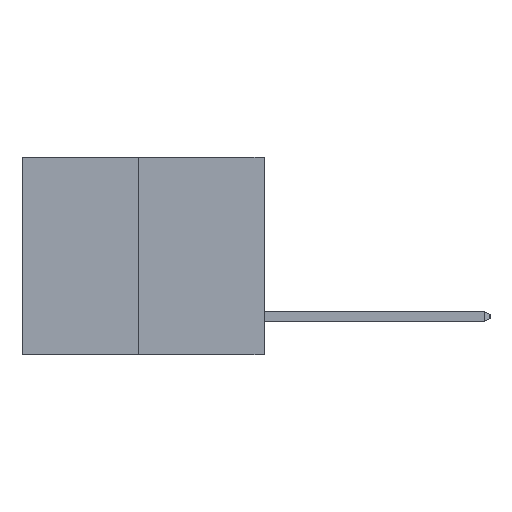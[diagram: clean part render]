
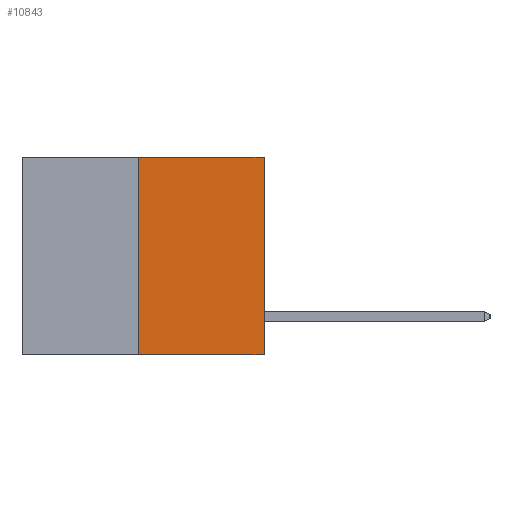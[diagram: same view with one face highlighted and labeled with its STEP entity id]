
A CAD part, left-side view. The second image highlights one B-rep face of the part: STEP entity #10843.
In plain terms, the highlighted planar face has unit normal (-1, 0, 0).
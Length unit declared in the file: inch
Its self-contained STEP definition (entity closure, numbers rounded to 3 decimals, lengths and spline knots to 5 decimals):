
#580 = LINE ( 'NONE', #10422, #9586 ) ;
#857 = CARTESIAN_POINT ( 'NONE',  ( 0., 0., 0. ) ) ;
#1157 = CARTESIAN_POINT ( 'NONE',  ( 0., 0.6, 0. ) ) ;
#1244 = CARTESIAN_POINT ( 'NONE',  ( 0., 0.312, -0.49 ) ) ;
#1453 = ORIENTED_EDGE ( 'NONE', *, *, #2829, .T. ) ;
#1583 = CARTESIAN_POINT ( 'NONE',  ( 0., 0., -0.49 ) ) ;
#1848 = FACE_OUTER_BOUND ( 'NONE', #2787, .T. ) ;
#2077 = CARTESIAN_POINT ( 'NONE',  ( 0., 0.6, -0.49 ) ) ;
#2404 = PLANE ( 'NONE',  #6178 ) ;
#2787 = EDGE_LOOP ( 'NONE', ( #13172, #1453, #3971, #11231 ) ) ;
#2829 = EDGE_CURVE ( 'NONE', #10470, #15645, #11234, .T. ) ;
#3025 = DIRECTION ( 'NONE',  ( 0., 0., 1. ) ) ;
#3500 = DIRECTION ( 'NONE',  ( 0., -1., 0. ) ) ;
#3876 = VERTEX_POINT ( 'NONE', #857 ) ;
#3971 = ORIENTED_EDGE ( 'NONE', *, *, #5435, .T. ) ;
#4559 = CARTESIAN_POINT ( 'NONE',  ( 0., 0.6, 0. ) ) ;
#5435 = EDGE_CURVE ( 'NONE', #15645, #3876, #580, .T. ) ;
#6178 = AXIS2_PLACEMENT_3D ( 'NONE', #1157, #14856, #16010 ) ;
#6462 = DIRECTION ( 'NONE',  ( 0., 0., 1. ) ) ;
#6846 = CARTESIAN_POINT ( 'NONE',  ( 0., 0.312, 0. ) ) ;
#7126 = CARTESIAN_POINT ( 'NONE',  ( 0., 0.312, -0.49 ) ) ;
#8089 = EDGE_CURVE ( 'NONE', #12696, #3876, #8664, .T. ) ;
#8664 = LINE ( 'NONE', #4559, #17399 ) ;
#9586 = VECTOR ( 'NONE', #6462, 39.37008 ) ;
#10257 = DIRECTION ( 'NONE',  ( 0., -1., 0. ) ) ;
#10382 = VECTOR ( 'NONE', #3500, 39.37008 ) ;
#10422 = CARTESIAN_POINT ( 'NONE',  ( 0., 0., 0. ) ) ;
#10470 = VERTEX_POINT ( 'NONE', #7126 ) ;
#10843 = ADVANCED_FACE ( 'NONE', ( #1848 ), #2404, .F. ) ;
#11231 = ORIENTED_EDGE ( 'NONE', *, *, #8089, .F. ) ;
#11234 = LINE ( 'NONE', #2077, #10382 ) ;
#12696 = VERTEX_POINT ( 'NONE', #6846 ) ;
#12871 = LINE ( 'NONE', #1244, #16032 ) ;
#13172 = ORIENTED_EDGE ( 'NONE', *, *, #14270, .F. ) ;
#14270 = EDGE_CURVE ( 'NONE', #10470, #12696, #12871, .T. ) ;
#14856 = DIRECTION ( 'NONE',  ( 1., 0., 0. ) ) ;
#15645 = VERTEX_POINT ( 'NONE', #1583 ) ;
#16010 = DIRECTION ( 'NONE',  ( 0., 0., -1. ) ) ;
#16032 = VECTOR ( 'NONE', #3025, 39.37008 ) ;
#17399 = VECTOR ( 'NONE', #10257, 39.37008 ) ;
